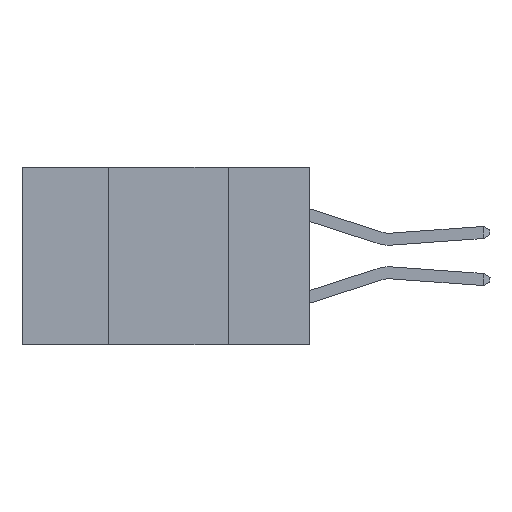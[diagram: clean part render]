
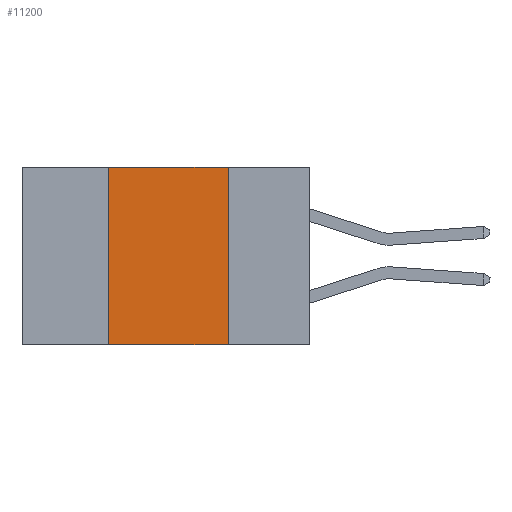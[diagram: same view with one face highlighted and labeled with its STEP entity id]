
A CAD part, left-side view. The second image highlights one B-rep face of the part: STEP entity #11200.
In plain terms, the highlighted planar face has unit normal (-1, 0, 0).
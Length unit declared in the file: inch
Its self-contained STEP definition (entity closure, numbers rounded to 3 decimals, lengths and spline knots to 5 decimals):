
#246 = DIRECTION ( 'NONE',  ( 0., 0., -1. ) ) ;
#269 = EDGE_CURVE ( 'NONE', #13284, #2882, #6130, .T. ) ;
#485 = CARTESIAN_POINT ( 'NONE',  ( 0., 0.17, -0.37 ) ) ;
#1164 = DIRECTION ( 'NONE',  ( 0., 0., 1. ) ) ;
#2175 = VECTOR ( 'NONE', #1164, 39.37008 ) ;
#2612 = VECTOR ( 'NONE', #11355, 39.37008 ) ;
#2882 = VERTEX_POINT ( 'NONE', #19391 ) ;
#3329 = PLANE ( 'NONE',  #6705 ) ;
#4507 = CARTESIAN_POINT ( 'NONE',  ( 0., 0.6, -0.37 ) ) ;
#6130 = LINE ( 'NONE', #485, #9641 ) ;
#6188 = VERTEX_POINT ( 'NONE', #13927 ) ;
#6414 = CARTESIAN_POINT ( 'NONE',  ( 0., 0.6, 0. ) ) ;
#6441 = EDGE_CURVE ( 'NONE', #8219, #13284, #14188, .T. ) ;
#6633 = EDGE_LOOP ( 'NONE', ( #10503, #6937, #11438, #15864 ) ) ;
#6705 = AXIS2_PLACEMENT_3D ( 'NONE', #6414, #9430, #246 ) ;
#6937 = ORIENTED_EDGE ( 'NONE', *, *, #6441, .F. ) ;
#8219 = VERTEX_POINT ( 'NONE', #11027 ) ;
#9430 = DIRECTION ( 'NONE',  ( 1., 0., 0. ) ) ;
#9562 = CARTESIAN_POINT ( 'NONE',  ( 0., 0.17, 0. ) ) ;
#9641 = VECTOR ( 'NONE', #11234, 39.37008 ) ;
#10503 = ORIENTED_EDGE ( 'NONE', *, *, #269, .F. ) ;
#10860 = FACE_OUTER_BOUND ( 'NONE', #6633, .T. ) ;
#11027 = CARTESIAN_POINT ( 'NONE',  ( 0., 0.42, 0. ) ) ;
#11200 = ADVANCED_FACE ( 'NONE', ( #10860 ), #3329, .F. ) ;
#11234 = DIRECTION ( 'NONE',  ( 0., 0., -1. ) ) ;
#11327 = CARTESIAN_POINT ( 'NONE',  ( 0., 0.6, 0. ) ) ;
#11355 = DIRECTION ( 'NONE',  ( 0., -1., 0. ) ) ;
#11438 = ORIENTED_EDGE ( 'NONE', *, *, #18510, .F. ) ;
#12393 = VECTOR ( 'NONE', #16527, 39.37008 ) ;
#12854 = LINE ( 'NONE', #4507, #12393 ) ;
#13284 = VERTEX_POINT ( 'NONE', #9562 ) ;
#13927 = CARTESIAN_POINT ( 'NONE',  ( 0., 0.42, -0.37 ) ) ;
#14188 = LINE ( 'NONE', #11327, #2612 ) ;
#14732 = LINE ( 'NONE', #19227, #2175 ) ;
#15864 = ORIENTED_EDGE ( 'NONE', *, *, #18630, .T. ) ;
#16527 = DIRECTION ( 'NONE',  ( 0., -1., 0. ) ) ;
#18510 = EDGE_CURVE ( 'NONE', #6188, #8219, #14732, .T. ) ;
#18630 = EDGE_CURVE ( 'NONE', #6188, #2882, #12854, .T. ) ;
#19227 = CARTESIAN_POINT ( 'NONE',  ( 0., 0.42, -0.37 ) ) ;
#19391 = CARTESIAN_POINT ( 'NONE',  ( 0., 0.17, -0.37 ) ) ;
